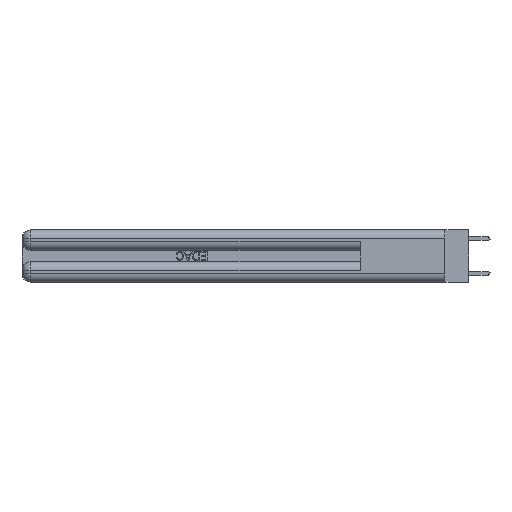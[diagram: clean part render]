
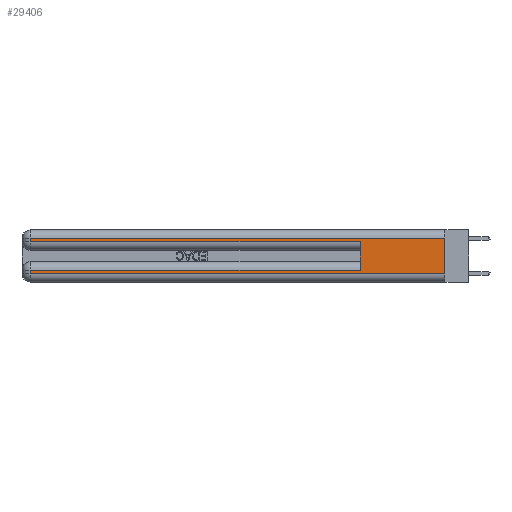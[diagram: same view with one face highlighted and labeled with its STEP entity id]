
A CAD part, left-side view. The second image highlights one B-rep face of the part: STEP entity #29406.
In plain terms, the highlighted planar face has unit normal (-1, 0, 0).
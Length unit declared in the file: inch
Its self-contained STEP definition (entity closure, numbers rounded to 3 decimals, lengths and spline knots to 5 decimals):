
#1122 = AXIS2_PLACEMENT_3D ( 'NONE', #21840, #10949, #23943 ) ;
#2433 = ORIENTED_EDGE ( 'NONE', *, *, #11675, .T. ) ;
#2436 = CARTESIAN_POINT ( 'NONE',  ( 0., 2.94, 0.37 ) ) ;
#2627 = DIRECTION ( 'NONE',  ( 0., -1., 0. ) ) ;
#3240 = VERTEX_POINT ( 'NONE', #27079 ) ;
#4113 = VERTEX_POINT ( 'NONE', #18379 ) ;
#4289 = EDGE_CURVE ( 'NONE', #8785, #21619, #33798, .T. ) ;
#4417 = CARTESIAN_POINT ( 'NONE',  ( 0., 0.6, 0.085 ) ) ;
#4452 = CARTESIAN_POINT ( 'NONE',  ( 0., 2.94, 0.31 ) ) ;
#5089 = VERTEX_POINT ( 'NONE', #27383 ) ;
#5234 = DIRECTION ( 'NONE',  ( 0., 0., -1. ) ) ;
#5256 = LINE ( 'NONE', #26705, #12536 ) ;
#6794 = CARTESIAN_POINT ( 'NONE',  ( 0., 0., 0.31 ) ) ;
#6806 = LINE ( 'NONE', #27896, #18443 ) ;
#6884 = VERTEX_POINT ( 'NONE', #4452 ) ;
#7053 = CARTESIAN_POINT ( 'NONE',  ( 0., 0., 0.085 ) ) ;
#7722 = ORIENTED_EDGE ( 'NONE', *, *, #27471, .F. ) ;
#8785 = VERTEX_POINT ( 'NONE', #4417 ) ;
#9269 = DIRECTION ( 'NONE',  ( 0., 1., 0. ) ) ;
#10486 = LINE ( 'NONE', #13843, #14453 ) ;
#10735 = EDGE_CURVE ( 'NONE', #3240, #4113, #5256, .T. ) ;
#10949 = DIRECTION ( 'NONE',  ( 1., 0., 0. ) ) ;
#11333 = DIRECTION ( 'NONE',  ( 0., 0., -1. ) ) ;
#11619 = CARTESIAN_POINT ( 'NONE',  ( 0., 2.94, 0.085 ) ) ;
#11675 = EDGE_CURVE ( 'NONE', #21619, #3240, #31289, .T. ) ;
#12021 = VERTEX_POINT ( 'NONE', #6794 ) ;
#12536 = VECTOR ( 'NONE', #2627, 39.37008 ) ;
#13601 = EDGE_CURVE ( 'NONE', #5089, #30589, #24015, .T. ) ;
#13843 = CARTESIAN_POINT ( 'NONE',  ( 0., 2.94, 0.37 ) ) ;
#14080 = ORIENTED_EDGE ( 'NONE', *, *, #26842, .T. ) ;
#14453 = VECTOR ( 'NONE', #24545, 39.37008 ) ;
#18242 = EDGE_CURVE ( 'NONE', #12021, #4113, #21677, .T. ) ;
#18379 = CARTESIAN_POINT ( 'NONE',  ( 0., 0., 0.06 ) ) ;
#18443 = VECTOR ( 'NONE', #9269, 39.37008 ) ;
#19239 = CARTESIAN_POINT ( 'NONE',  ( 0., 0.6, 0.145 ) ) ;
#19979 = VECTOR ( 'NONE', #32824, 39.37008 ) ;
#20009 = VECTOR ( 'NONE', #11333, 39.37008 ) ;
#21619 = VERTEX_POINT ( 'NONE', #11619 ) ;
#21677 = LINE ( 'NONE', #25017, #20009 ) ;
#21840 = CARTESIAN_POINT ( 'NONE',  ( 0., 0., 0.37 ) ) ;
#22102 = CARTESIAN_POINT ( 'NONE',  ( 0., 0., 0.285 ) ) ;
#22808 = ORIENTED_EDGE ( 'NONE', *, *, #34022, .T. ) ;
#23065 = ORIENTED_EDGE ( 'NONE', *, *, #10735, .T. ) ;
#23561 = VECTOR ( 'NONE', #27145, 39.37008 ) ;
#23943 = DIRECTION ( 'NONE',  ( 0., 0., -1. ) ) ;
#23976 = LINE ( 'NONE', #19239, #23561 ) ;
#24015 = LINE ( 'NONE', #22102, #19979 ) ;
#24180 = ORIENTED_EDGE ( 'NONE', *, *, #13601, .T. ) ;
#24373 = ORIENTED_EDGE ( 'NONE', *, *, #4289, .T. ) ;
#24545 = DIRECTION ( 'NONE',  ( 0., 0., -1. ) ) ;
#25017 = CARTESIAN_POINT ( 'NONE',  ( 0., 0., 0.37 ) ) ;
#26053 = CARTESIAN_POINT ( 'NONE',  ( 0., 0.6, 0.285 ) ) ;
#26476 = VECTOR ( 'NONE', #31158, 39.37008 ) ;
#26705 = CARTESIAN_POINT ( 'NONE',  ( 0., 0., 0.06 ) ) ;
#26842 = EDGE_CURVE ( 'NONE', #6884, #5089, #10486, .T. ) ;
#26927 = PLANE ( 'NONE',  #1122 ) ;
#27079 = CARTESIAN_POINT ( 'NONE',  ( 0., 2.94, 0.06 ) ) ;
#27145 = DIRECTION ( 'NONE',  ( 0., 0., 1. ) ) ;
#27383 = CARTESIAN_POINT ( 'NONE',  ( 0., 2.94, 0.285 ) ) ;
#27471 = EDGE_CURVE ( 'NONE', #8785, #30589, #23976, .T. ) ;
#27896 = CARTESIAN_POINT ( 'NONE',  ( 0., 0., 0.31 ) ) ;
#28354 = ORIENTED_EDGE ( 'NONE', *, *, #18242, .F. ) ;
#28754 = VECTOR ( 'NONE', #5234, 39.37008 ) ;
#29406 = ADVANCED_FACE ( 'NONE', ( #32399 ), #26927, .F. ) ;
#30589 = VERTEX_POINT ( 'NONE', #26053 ) ;
#31158 = DIRECTION ( 'NONE',  ( 0., 1., 0. ) ) ;
#31289 = LINE ( 'NONE', #2436, #28754 ) ;
#32399 = FACE_OUTER_BOUND ( 'NONE', #33021, .T. ) ;
#32824 = DIRECTION ( 'NONE',  ( 0., -1., 0. ) ) ;
#33021 = EDGE_LOOP ( 'NONE', ( #28354, #22808, #14080, #24180, #7722, #24373, #2433, #23065 ) ) ;
#33798 = LINE ( 'NONE', #7053, #26476 ) ;
#34022 = EDGE_CURVE ( 'NONE', #12021, #6884, #6806, .T. ) ;
